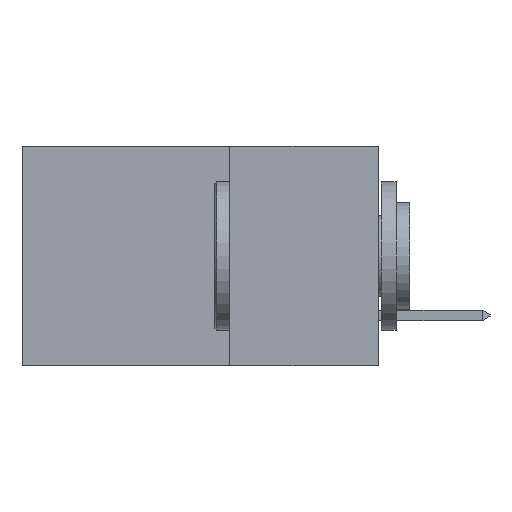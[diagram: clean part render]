
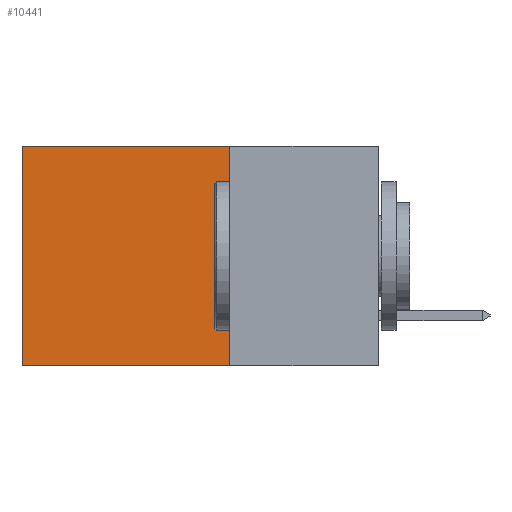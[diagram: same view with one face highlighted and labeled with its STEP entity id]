
A CAD part, left-side view. The second image highlights one B-rep face of the part: STEP entity #10441.
In plain terms, the highlighted planar face has unit normal (-1, 0, 0).
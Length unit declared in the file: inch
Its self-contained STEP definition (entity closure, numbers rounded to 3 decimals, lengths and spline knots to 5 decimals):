
#247 = VECTOR ( 'NONE', #19377, 39.37008 ) ;
#556 = CARTESIAN_POINT ( 'NONE',  ( 0.298, 0.25, 0. ) ) ;
#867 = EDGE_CURVE ( 'NONE', #9447, #23920, #6937, .T. ) ;
#1104 = CARTESIAN_POINT ( 'NONE',  ( 0.298, 0.25, 0. ) ) ;
#1835 = EDGE_LOOP ( 'NONE', ( #22217, #8212, #13530, #13245 ) ) ;
#1841 = AXIS2_PLACEMENT_3D ( 'NONE', #17774, #19605, #8543 ) ;
#1876 = VECTOR ( 'NONE', #1944, 39.37008 ) ;
#1944 = DIRECTION ( 'NONE',  ( 0., 0., -1. ) ) ;
#2595 = CARTESIAN_POINT ( 'NONE',  ( 0.298, 0.6, 0. ) ) ;
#5302 = LINE ( 'NONE', #2595, #247 ) ;
#5384 = CARTESIAN_POINT ( 'NONE',  ( 0.298, 0.25, 0. ) ) ;
#6412 = CARTESIAN_POINT ( 'NONE',  ( 0.298, 0.6, -0.37 ) ) ;
#6898 = EDGE_CURVE ( 'NONE', #20815, #10347, #5302, .T. ) ;
#6937 = LINE ( 'NONE', #1104, #1876 ) ;
#7267 = DIRECTION ( 'NONE',  ( 0., 1., 0. ) ) ;
#8212 = ORIENTED_EDGE ( 'NONE', *, *, #22281, .F. ) ;
#8543 = DIRECTION ( 'NONE',  ( 0., 0., -1. ) ) ;
#9447 = VERTEX_POINT ( 'NONE', #556 ) ;
#10347 = VERTEX_POINT ( 'NONE', #6412 ) ;
#10441 = ADVANCED_FACE ( 'NONE', ( #17342 ), #14035, .F. ) ;
#10834 = LINE ( 'NONE', #19077, #20036 ) ;
#11751 = VECTOR ( 'NONE', #7267, 39.37008 ) ;
#12351 = LINE ( 'NONE', #5384, #11751 ) ;
#13245 = ORIENTED_EDGE ( 'NONE', *, *, #22024, .T. ) ;
#13530 = ORIENTED_EDGE ( 'NONE', *, *, #867, .F. ) ;
#14035 = PLANE ( 'NONE',  #1841 ) ;
#17272 = DIRECTION ( 'NONE',  ( 0., 1., 0. ) ) ;
#17342 = FACE_OUTER_BOUND ( 'NONE', #1835, .T. ) ;
#17774 = CARTESIAN_POINT ( 'NONE',  ( 0.298, 0.25, 0. ) ) ;
#19077 = CARTESIAN_POINT ( 'NONE',  ( 0.298, 0.25, -0.37 ) ) ;
#19340 = CARTESIAN_POINT ( 'NONE',  ( 0.298, 0.6, 0. ) ) ;
#19377 = DIRECTION ( 'NONE',  ( 0., 0., -1. ) ) ;
#19605 = DIRECTION ( 'NONE',  ( 1., 0., 0. ) ) ;
#20036 = VECTOR ( 'NONE', #17272, 39.37008 ) ;
#20815 = VERTEX_POINT ( 'NONE', #19340 ) ;
#22024 = EDGE_CURVE ( 'NONE', #9447, #20815, #12351, .T. ) ;
#22058 = CARTESIAN_POINT ( 'NONE',  ( 0.298, 0.25, -0.37 ) ) ;
#22217 = ORIENTED_EDGE ( 'NONE', *, *, #6898, .T. ) ;
#22281 = EDGE_CURVE ( 'NONE', #23920, #10347, #10834, .T. ) ;
#23920 = VERTEX_POINT ( 'NONE', #22058 ) ;
